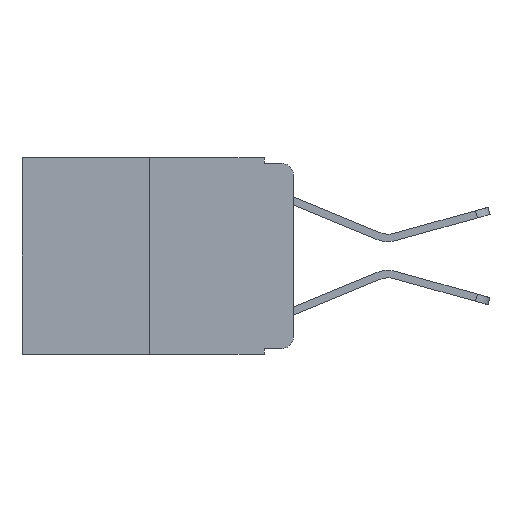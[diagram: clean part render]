
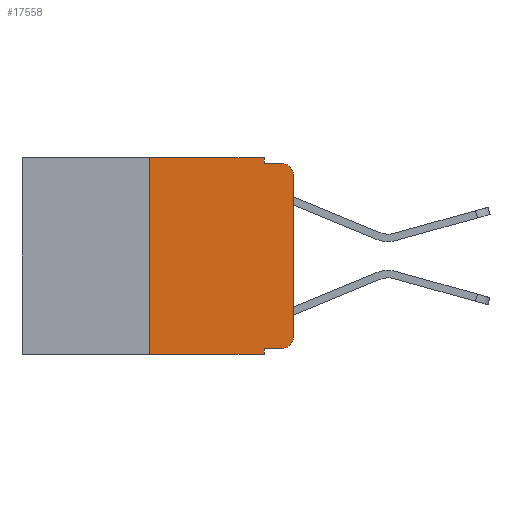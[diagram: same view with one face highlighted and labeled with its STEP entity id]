
A CAD part, left-side view. The second image highlights one B-rep face of the part: STEP entity #17558.
In plain terms, the highlighted planar face has unit normal (-1, 0, 0).
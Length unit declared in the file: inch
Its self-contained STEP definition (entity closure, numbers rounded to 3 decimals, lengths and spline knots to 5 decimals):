
#544 = CARTESIAN_POINT ( 'NONE',  ( 0., 0., 0. ) ) ;
#772 = VERTEX_POINT ( 'NONE', #6317 ) ;
#1059 = DIRECTION ( 'NONE',  ( 0., -1., 0. ) ) ;
#1397 = CARTESIAN_POINT ( 'NONE',  ( 0., 0.02, -0.313 ) ) ;
#1431 = DIRECTION ( 'NONE',  ( 0., 0., -1. ) ) ;
#1539 = LINE ( 'NONE', #5803, #8848 ) ;
#1648 = CARTESIAN_POINT ( 'NONE',  ( 0., 0.051, 0. ) ) ;
#1710 = CIRCLE ( 'NONE', #2594, 0.02 ) ;
#1735 = VECTOR ( 'NONE', #13338, 39.37008 ) ;
#1924 = CARTESIAN_POINT ( 'NONE',  ( 0., 0.473, -0.343 ) ) ;
#2260 = CARTESIAN_POINT ( 'NONE',  ( 0., 0.051, 0. ) ) ;
#2299 = VECTOR ( 'NONE', #8724, 39.37008 ) ;
#2594 = AXIS2_PLACEMENT_3D ( 'NONE', #1397, #16774, #16508 ) ;
#3347 = EDGE_CURVE ( 'NONE', #3747, #3371, #9635, .T. ) ;
#3371 = VERTEX_POINT ( 'NONE', #12679 ) ;
#3723 = ORIENTED_EDGE ( 'NONE', *, *, #5741, .T. ) ;
#3747 = VERTEX_POINT ( 'NONE', #15395 ) ;
#3799 = EDGE_CURVE ( 'NONE', #8594, #16228, #6592, .T. ) ;
#4470 = VECTOR ( 'NONE', #1059, 39.37008 ) ;
#4626 = VECTOR ( 'NONE', #12123, 39.37008 ) ;
#4656 = DIRECTION ( 'NONE',  ( 0., 0., -1. ) ) ;
#5177 = CARTESIAN_POINT ( 'NONE',  ( 0., 0.051, -0.333 ) ) ;
#5551 = AXIS2_PLACEMENT_3D ( 'NONE', #15524, #8513, #1431 ) ;
#5622 = LINE ( 'NONE', #16371, #17772 ) ;
#5644 = CARTESIAN_POINT ( 'NONE',  ( 0., 0.051, -0.333 ) ) ;
#5688 = EDGE_CURVE ( 'NONE', #14290, #12008, #8829, .T. ) ;
#5706 = ORIENTED_EDGE ( 'NONE', *, *, #5688, .F. ) ;
#5741 = EDGE_CURVE ( 'NONE', #772, #12008, #14713, .T. ) ;
#5774 = VERTEX_POINT ( 'NONE', #13437 ) ;
#5803 = CARTESIAN_POINT ( 'NONE',  ( 0., 0.051, -0.01 ) ) ;
#6317 = CARTESIAN_POINT ( 'NONE',  ( 0., 0.25, -0.343 ) ) ;
#6592 = LINE ( 'NONE', #13501, #4470 ) ;
#6804 = ORIENTED_EDGE ( 'NONE', *, *, #10936, .T. ) ;
#6895 = DIRECTION ( 'NONE',  ( 0., -1., 0. ) ) ;
#7443 = LINE ( 'NONE', #544, #12508 ) ;
#7818 = ORIENTED_EDGE ( 'NONE', *, *, #3799, .F. ) ;
#7951 = LINE ( 'NONE', #11850, #4626 ) ;
#8078 = ORIENTED_EDGE ( 'NONE', *, *, #13517, .T. ) ;
#8150 = ORIENTED_EDGE ( 'NONE', *, *, #17330, .F. ) ;
#8392 = CARTESIAN_POINT ( 'NONE',  ( 0., 0.473, 0. ) ) ;
#8501 = ORIENTED_EDGE ( 'NONE', *, *, #3347, .T. ) ;
#8513 = DIRECTION ( 'NONE',  ( -1., 0., 0. ) ) ;
#8594 = VERTEX_POINT ( 'NONE', #11691 ) ;
#8724 = DIRECTION ( 'NONE',  ( 0., -1., 0. ) ) ;
#8829 = LINE ( 'NONE', #2260, #15384 ) ;
#8848 = VECTOR ( 'NONE', #6895, 39.37008 ) ;
#9593 = EDGE_LOOP ( 'NONE', ( #11823, #8501, #11805, #8150, #7818, #11110, #3723, #5706, #6804, #8078 ) ) ;
#9635 = CIRCLE ( 'NONE', #5551, 0.02 ) ;
#10032 = EDGE_CURVE ( 'NONE', #10837, #3747, #7443, .T. ) ;
#10223 = EDGE_CURVE ( 'NONE', #772, #8594, #5622, .T. ) ;
#10679 = CARTESIAN_POINT ( 'NONE',  ( 0., 0.02, -0.333 ) ) ;
#10837 = VERTEX_POINT ( 'NONE', #17765 ) ;
#10936 = EDGE_CURVE ( 'NONE', #14290, #14790, #11448, .T. ) ;
#11016 = AXIS2_PLACEMENT_3D ( 'NONE', #8392, #16509, #11212 ) ;
#11085 = DIRECTION ( 'NONE',  ( 0., 0., 1. ) ) ;
#11110 = ORIENTED_EDGE ( 'NONE', *, *, #10223, .F. ) ;
#11212 = DIRECTION ( 'NONE',  ( 0., 0., -1. ) ) ;
#11448 = LINE ( 'NONE', #5644, #2299 ) ;
#11691 = CARTESIAN_POINT ( 'NONE',  ( 0., 0.25, 0. ) ) ;
#11805 = ORIENTED_EDGE ( 'NONE', *, *, #15318, .F. ) ;
#11823 = ORIENTED_EDGE ( 'NONE', *, *, #10032, .T. ) ;
#11850 = CARTESIAN_POINT ( 'NONE',  ( 0., 0.051, 0. ) ) ;
#12008 = VERTEX_POINT ( 'NONE', #13489 ) ;
#12123 = DIRECTION ( 'NONE',  ( 0., 0., -1. ) ) ;
#12508 = VECTOR ( 'NONE', #17194, 39.37008 ) ;
#12679 = CARTESIAN_POINT ( 'NONE',  ( 0., 0.02, -0.01 ) ) ;
#13338 = DIRECTION ( 'NONE',  ( 0., -1., 0. ) ) ;
#13437 = CARTESIAN_POINT ( 'NONE',  ( 0., 0.051, -0.01 ) ) ;
#13489 = CARTESIAN_POINT ( 'NONE',  ( 0., 0.051, -0.343 ) ) ;
#13501 = CARTESIAN_POINT ( 'NONE',  ( 0., 0.473, 0. ) ) ;
#13517 = EDGE_CURVE ( 'NONE', #14790, #10837, #1710, .T. ) ;
#14026 = PLANE ( 'NONE',  #11016 ) ;
#14290 = VERTEX_POINT ( 'NONE', #5177 ) ;
#14713 = LINE ( 'NONE', #1924, #1735 ) ;
#14790 = VERTEX_POINT ( 'NONE', #10679 ) ;
#15318 = EDGE_CURVE ( 'NONE', #5774, #3371, #1539, .T. ) ;
#15384 = VECTOR ( 'NONE', #4656, 39.37008 ) ;
#15395 = CARTESIAN_POINT ( 'NONE',  ( 0., 0., -0.03 ) ) ;
#15499 = FACE_OUTER_BOUND ( 'NONE', #9593, .T. ) ;
#15524 = CARTESIAN_POINT ( 'NONE',  ( 0., 0.02, -0.03 ) ) ;
#16228 = VERTEX_POINT ( 'NONE', #1648 ) ;
#16371 = CARTESIAN_POINT ( 'NONE',  ( 0., 0.25, 0. ) ) ;
#16508 = DIRECTION ( 'NONE',  ( 0., 0., -1. ) ) ;
#16509 = DIRECTION ( 'NONE',  ( 1., 0., 0. ) ) ;
#16774 = DIRECTION ( 'NONE',  ( -1., 0., 0. ) ) ;
#17194 = DIRECTION ( 'NONE',  ( 0., 0., 1. ) ) ;
#17330 = EDGE_CURVE ( 'NONE', #16228, #5774, #7951, .T. ) ;
#17558 = ADVANCED_FACE ( 'NONE', ( #15499 ), #14026, .F. ) ;
#17765 = CARTESIAN_POINT ( 'NONE',  ( 0., 0., -0.313 ) ) ;
#17772 = VECTOR ( 'NONE', #11085, 39.37008 ) ;
